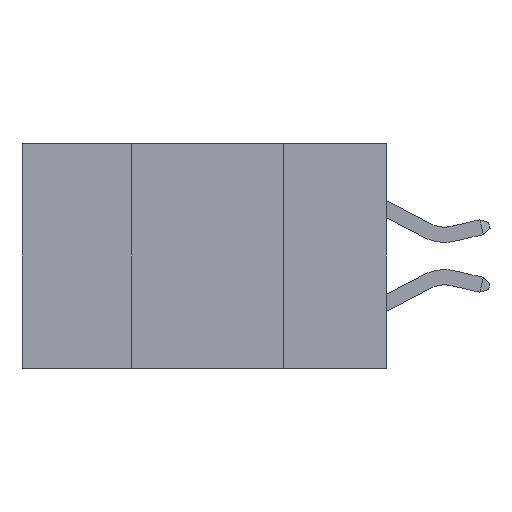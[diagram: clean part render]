
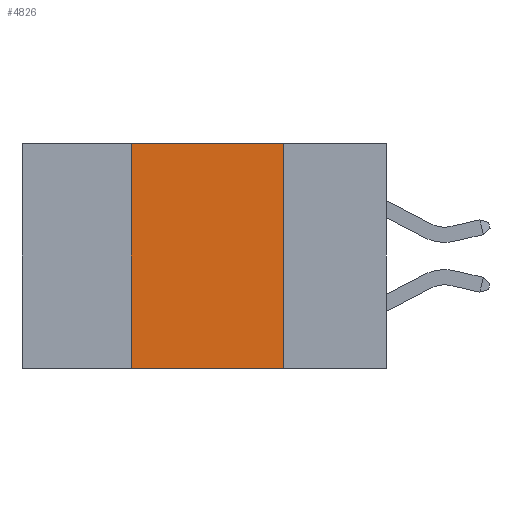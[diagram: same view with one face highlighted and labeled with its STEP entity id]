
A CAD part, left-side view. The second image highlights one B-rep face of the part: STEP entity #4826.
In plain terms, the highlighted planar face has unit normal (-1, 0, 0).
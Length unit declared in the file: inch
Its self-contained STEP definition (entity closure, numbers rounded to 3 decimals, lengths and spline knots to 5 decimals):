
#20 = FACE_OUTER_BOUND ( 'NONE', #4030, .T. ) ;
#197 = CARTESIAN_POINT ( 'NONE',  ( 0., 0.17, -0.37 ) ) ;
#218 = LINE ( 'NONE', #23722, #19265 ) ;
#696 = EDGE_CURVE ( 'NONE', #14336, #3268, #23483, .T. ) ;
#822 = CARTESIAN_POINT ( 'NONE',  ( 0., 0.17, 0. ) ) ;
#835 = EDGE_CURVE ( 'NONE', #3268, #18789, #218, .T. ) ;
#1793 = CARTESIAN_POINT ( 'NONE',  ( 0., 0.6, 0. ) ) ;
#1858 = CARTESIAN_POINT ( 'NONE',  ( 0., 0.6, 0. ) ) ;
#3268 = VERTEX_POINT ( 'NONE', #822 ) ;
#3533 = AXIS2_PLACEMENT_3D ( 'NONE', #1793, #13494, #13238 ) ;
#4030 = EDGE_LOOP ( 'NONE', ( #22854, #23079, #6506, #11158 ) ) ;
#4802 = VERTEX_POINT ( 'NONE', #17259 ) ;
#4826 = ADVANCED_FACE ( 'NONE', ( #20 ), #15132, .F. ) ;
#4852 = DIRECTION ( 'NONE',  ( 0., 0., -1. ) ) ;
#5429 = CARTESIAN_POINT ( 'NONE',  ( 0., 0.6, -0.37 ) ) ;
#6045 = DIRECTION ( 'NONE',  ( 0., 0., 1. ) ) ;
#6506 = ORIENTED_EDGE ( 'NONE', *, *, #15236, .F. ) ;
#7197 = VECTOR ( 'NONE', #13108, 39.37008 ) ;
#7330 = LINE ( 'NONE', #5429, #7197 ) ;
#7940 = CARTESIAN_POINT ( 'NONE',  ( 0., 0.42, -0.37 ) ) ;
#9786 = DIRECTION ( 'NONE',  ( 0., -1., 0. ) ) ;
#11158 = ORIENTED_EDGE ( 'NONE', *, *, #22659, .T. ) ;
#11721 = LINE ( 'NONE', #7940, #12094 ) ;
#12094 = VECTOR ( 'NONE', #6045, 39.37008 ) ;
#13108 = DIRECTION ( 'NONE',  ( 0., -1., 0. ) ) ;
#13238 = DIRECTION ( 'NONE',  ( 0., 0., -1. ) ) ;
#13494 = DIRECTION ( 'NONE',  ( 1., 0., 0. ) ) ;
#14336 = VERTEX_POINT ( 'NONE', #23044 ) ;
#15132 = PLANE ( 'NONE',  #3533 ) ;
#15236 = EDGE_CURVE ( 'NONE', #4802, #14336, #11721, .T. ) ;
#17259 = CARTESIAN_POINT ( 'NONE',  ( 0., 0.42, -0.37 ) ) ;
#18789 = VERTEX_POINT ( 'NONE', #197 ) ;
#19265 = VECTOR ( 'NONE', #4852, 39.37008 ) ;
#22478 = VECTOR ( 'NONE', #9786, 39.37008 ) ;
#22659 = EDGE_CURVE ( 'NONE', #4802, #18789, #7330, .T. ) ;
#22854 = ORIENTED_EDGE ( 'NONE', *, *, #835, .F. ) ;
#23044 = CARTESIAN_POINT ( 'NONE',  ( 0., 0.42, 0. ) ) ;
#23079 = ORIENTED_EDGE ( 'NONE', *, *, #696, .F. ) ;
#23483 = LINE ( 'NONE', #1858, #22478 ) ;
#23722 = CARTESIAN_POINT ( 'NONE',  ( 0., 0.17, -0.37 ) ) ;
